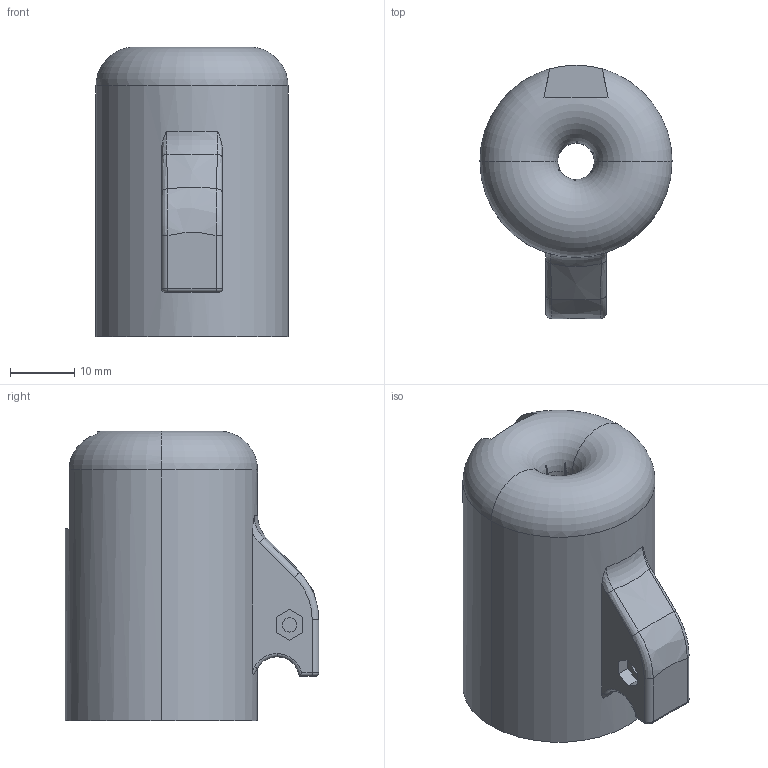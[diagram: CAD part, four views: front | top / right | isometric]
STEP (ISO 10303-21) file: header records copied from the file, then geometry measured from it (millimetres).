
FILE_DESCRIPTION (( 'STEP AP214' ), '1' );
FILE_NAME ('Barrel_.22_LR.step', '2013-11-06T14:30:33', ( 'elpi' ), ( '' ), 'SwSTEP 2.0', 'SolidWorks 2013', '' );
FILE_SCHEMA (( 'AUTOMOTIVE_DESIGN' ));
Length unit declared in the file: millimetre
Products named in the file (1): Barrel_.22_LR
Bounding box: 30 x 39.54 x 45.25 mm (x, y, z)
Volume: 30769.6 mm3; surface area: 6879.6 mm2
Topology: 1 solids, 1 shells, 155 faces, 360 edges, 212 vertices
Faces by surface type: bspline 79, plane 32, cylinder 20, torus 17, sphere 6, cone 1
Entity records: 7521 total; most frequent: CARTESIAN_POINT 4503, ORIENTED_EDGE 720, DIRECTION 492, EDGE_CURVE 360, VERTEX_POINT 212, AXIS2_PLACEMENT_3D 211, EDGE_LOOP 162, B_SPLINE_CURVE_WITH_KNOTS 156
